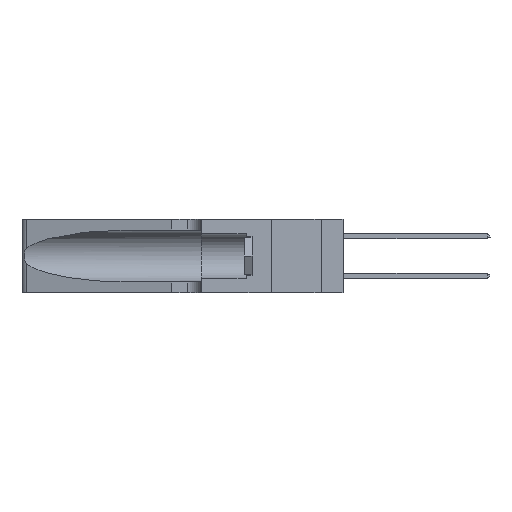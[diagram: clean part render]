
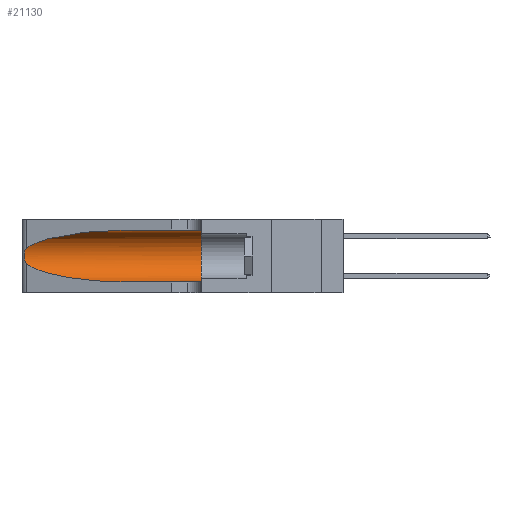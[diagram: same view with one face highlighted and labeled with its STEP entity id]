
A CAD part, left-side view. The second image highlights one B-rep face of the part: STEP entity #21130.
In plain terms, the highlighted cylindrical face has radius 3.308 mm (diameter 6.617 mm), a partial arc.
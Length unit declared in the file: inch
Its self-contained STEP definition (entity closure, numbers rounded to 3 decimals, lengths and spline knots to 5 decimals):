
#520 = CARTESIAN_POINT ( 'NONE',  ( 0.25487, 1.22718, 0.22369 ) ) ;
#597 = CARTESIAN_POINT ( 'NONE',  ( 0.25487, 1.22718, 0.22369 ) ) ;
#684 = CARTESIAN_POINT ( 'NONE',  ( 0.25787, 1.23484, 0.2124 ) ) ;
#1007 = DIRECTION ( 'NONE',  ( 0., -1., 0. ) ) ;
#1765 = ORIENTED_EDGE ( 'NONE', *, *, #2859, .T. ) ;
#2191 = EDGE_LOOP ( 'NONE', ( #1765, #9127, #2666, #21358, #15339, #19499 ) ) ;
#2269 = CARTESIAN_POINT ( 'NONE',  ( 0.2373, 1.15595, 0.08982 ) ) ;
#2573 = CARTESIAN_POINT ( 'NONE',  ( 0.26018, 1.23835, 0.19895 ) ) ;
#2666 = ORIENTED_EDGE ( 'NONE', *, *, #21841, .T. ) ;
#2859 = EDGE_CURVE ( 'NONE', #17030, #14860, #4610, .T. ) ;
#3421 = AXIS2_PLACEMENT_3D ( 'NONE', #9609, #5903, #22538 ) ;
#3597 = CARTESIAN_POINT ( 'NONE',  ( 0.18966, 0.96281, 0.31525 ) ) ;
#4023 = AXIS2_PLACEMENT_3D ( 'NONE', #15509, #4380, #17351 ) ;
#4380 = DIRECTION ( 'NONE',  ( 0., 1., 0. ) ) ;
#4455 = CARTESIAN_POINT ( 'NONE',  ( 0.26075, 1.23896, 0.178 ) ) ;
#4482 = VERTEX_POINT ( 'NONE', #10125 ) ;
#4610 =( BOUNDED_CURVE ( )  B_SPLINE_CURVE ( 3, ( #9195, #3597, #7371, #22126 ),
 .UNSPECIFIED., .F., .T. ) 
 B_SPLINE_CURVE_WITH_KNOTS ( ( 4, 4 ),
 ( 1.5708, 2.84003 ),
 .UNSPECIFIED. ) 
 CURVE ( )  GEOMETRIC_REPRESENTATION_ITEM ( )  RATIONAL_B_SPLINE_CURVE ( ( 1., 0.87, 0.87, 1. ) ) 
 REPRESENTATION_ITEM ( '' )  );
#5903 = DIRECTION ( 'NONE',  ( 0., -1., 0. ) ) ;
#6041 = CARTESIAN_POINT ( 'NONE',  ( 0.18966, 0.96281, 0.05475 ) ) ;
#6346 = CARTESIAN_POINT ( 'NONE',  ( 0.25856, 1.23593, 0.16098 ) ) ;
#7049 = VECTOR ( 'NONE', #23127, 39.37008 ) ;
#7070 = CARTESIAN_POINT ( 'NONE',  ( 0.25487, 1.22718, 0.14631 ) ) ;
#7371 = CARTESIAN_POINT ( 'NONE',  ( 0.2373, 1.15595, 0.28018 ) ) ;
#7674 = EDGE_CURVE ( 'NONE', #19365, #4482, #11963, .T. ) ;
#8208 = CARTESIAN_POINT ( 'NONE',  ( 0.25639, 1.23186, 0.15144 ) ) ;
#9127 = ORIENTED_EDGE ( 'NONE', *, *, #22470, .T. ) ;
#9195 = CARTESIAN_POINT ( 'NONE',  ( 0.1305, 0.72297, 0.31525 ) ) ;
#9561 = CIRCLE ( 'NONE', #4023, 0.13025 ) ;
#9609 = CARTESIAN_POINT ( 'NONE',  ( 0.1305, 1.61858, 0.185 ) ) ;
#9908 = FACE_OUTER_BOUND ( 'NONE', #2191, .T. ) ;
#10062 = VECTOR ( 'NONE', #1007, 39.37008 ) ;
#10066 = CARTESIAN_POINT ( 'NONE',  ( 0.25487, 1.22718, 0.14631 ) ) ;
#10125 = CARTESIAN_POINT ( 'NONE',  ( 0.1305, 0.35, 0.05475 ) ) ;
#10669 = LINE ( 'NONE', #23137, #10062 ) ;
#11588 = EDGE_CURVE ( 'NONE', #17030, #23170, #10669, .T. ) ;
#11864 = CARTESIAN_POINT ( 'NONE',  ( 0.25639, 1.23184, 0.21858 ) ) ;
#11963 = LINE ( 'NONE', #23045, #7049 ) ;
#13725 = CARTESIAN_POINT ( 'NONE',  ( 0.25854, 1.2359, 0.20912 ) ) ;
#13796 = B_SPLINE_CURVE_WITH_KNOTS ( 'NONE', 3,
 ( #597, #21060, #11864, #684, #13725, #2573, #15578, #4455, #17420, #6346, #19272, #8208, #21137, #10066 ),
 .UNSPECIFIED., .F., .F.,
 ( 4, 2, 2, 2, 2, 2, 4 ),
 ( 0., 0.00027, 0.00053, 0.00107, 0.0016, 0.00187, 0.00214 ),
 .UNSPECIFIED. ) ;
#14860 = VERTEX_POINT ( 'NONE', #520 ) ;
#14886 = EDGE_CURVE ( 'NONE', #23170, #4482, #9561, .T. ) ;
#15292 = CARTESIAN_POINT ( 'NONE',  ( 0.25487, 1.22718, 0.14631 ) ) ;
#15339 = ORIENTED_EDGE ( 'NONE', *, *, #14886, .F. ) ;
#15509 = CARTESIAN_POINT ( 'NONE',  ( 0.1305, 0.35, 0.185 ) ) ;
#15578 = CARTESIAN_POINT ( 'NONE',  ( 0.26075, 1.23896, 0.19203 ) ) ;
#16590 = CARTESIAN_POINT ( 'NONE',  ( 0.1305, 0.72297, 0.05475 ) ) ;
#16679 = CARTESIAN_POINT ( 'NONE',  ( 0.1305, 0.35, 0.31525 ) ) ;
#17030 = VERTEX_POINT ( 'NONE', #22717 ) ;
#17351 = DIRECTION ( 'NONE',  ( 0., 0., 1. ) ) ;
#17368 = VERTEX_POINT ( 'NONE', #7070 ) ;
#17420 = CARTESIAN_POINT ( 'NONE',  ( 0.26017, 1.23833, 0.17102 ) ) ;
#18979 = CARTESIAN_POINT ( 'NONE',  ( 0.1305, 0.72297, 0.05475 ) ) ;
#19272 = CARTESIAN_POINT ( 'NONE',  ( 0.25789, 1.23486, 0.15765 ) ) ;
#19365 = VERTEX_POINT ( 'NONE', #16590 ) ;
#19499 = ORIENTED_EDGE ( 'NONE', *, *, #11588, .F. ) ;
#21060 = CARTESIAN_POINT ( 'NONE',  ( 0.25555, 1.22994, 0.2215 ) ) ;
#21130 = ADVANCED_FACE ( 'NONE', ( #9908 ), #22420, .F. ) ;
#21137 = CARTESIAN_POINT ( 'NONE',  ( 0.25555, 1.22993, 0.14849 ) ) ;
#21358 = ORIENTED_EDGE ( 'NONE', *, *, #7674, .T. ) ;
#21841 = EDGE_CURVE ( 'NONE', #17368, #19365, #22850, .T. ) ;
#22126 = CARTESIAN_POINT ( 'NONE',  ( 0.25487, 1.22718, 0.22369 ) ) ;
#22420 = CYLINDRICAL_SURFACE ( 'NONE', #3421, 0.13025 ) ;
#22470 = EDGE_CURVE ( 'NONE', #14860, #17368, #13796, .T. ) ;
#22538 = DIRECTION ( 'NONE',  ( 0., 0., -1. ) ) ;
#22717 = CARTESIAN_POINT ( 'NONE',  ( 0.1305, 0.72297, 0.31525 ) ) ;
#22850 =( BOUNDED_CURVE ( )  B_SPLINE_CURVE ( 3, ( #15292, #2269, #6041, #18979 ),
 .UNSPECIFIED., .F., .F. ) 
 B_SPLINE_CURVE_WITH_KNOTS ( ( 4, 4 ),
 ( 3.44316, 4.71239 ),
 .UNSPECIFIED. ) 
 CURVE ( )  GEOMETRIC_REPRESENTATION_ITEM ( )  RATIONAL_B_SPLINE_CURVE ( ( 1., 0.87, 0.87, 1. ) ) 
 REPRESENTATION_ITEM ( '' )  );
#23045 = CARTESIAN_POINT ( 'NONE',  ( 0.1305, 1.61858, 0.05475 ) ) ;
#23127 = DIRECTION ( 'NONE',  ( 0., -1., 0. ) ) ;
#23137 = CARTESIAN_POINT ( 'NONE',  ( 0.1305, 1.61858, 0.31525 ) ) ;
#23170 = VERTEX_POINT ( 'NONE', #16679 ) ;
